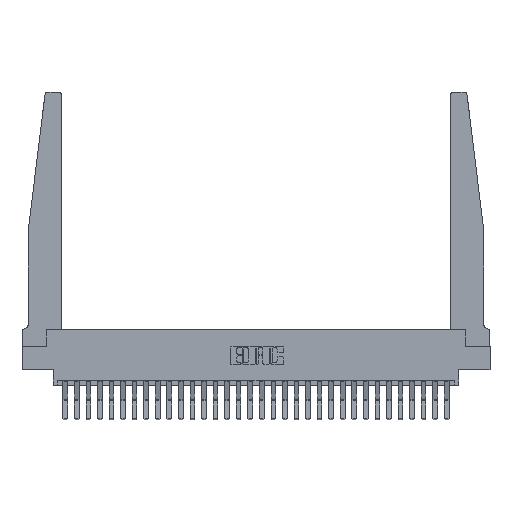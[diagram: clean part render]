
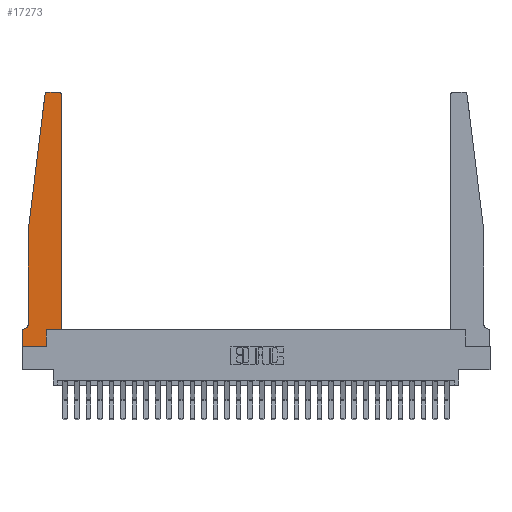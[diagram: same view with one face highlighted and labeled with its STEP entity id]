
A CAD part, top view. The second image highlights one B-rep face of the part: STEP entity #17273.
In plain terms, the highlighted planar face has unit normal (0, 0, 1).
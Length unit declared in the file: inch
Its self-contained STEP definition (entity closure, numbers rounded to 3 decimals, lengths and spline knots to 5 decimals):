
#343 = DIRECTION ( 'NONE',  ( 0., 0., 1. ) ) ;
#1655 = LINE ( 'NONE', #13245, #10600 ) ;
#1844 = LINE ( 'NONE', #19845, #6738 ) ;
#1891 = ORIENTED_EDGE ( 'NONE', *, *, #9325, .T. ) ;
#1930 = DIRECTION ( 'NONE',  ( 0., 0., 1. ) ) ;
#2151 = VERTEX_POINT ( 'NONE', #14245 ) ;
#2235 = VERTEX_POINT ( 'NONE', #6122 ) ;
#2693 = CARTESIAN_POINT ( 'NONE',  ( 0.2605, 0., 0.37 ) ) ;
#2800 = LINE ( 'NONE', #15864, #24524 ) ;
#2939 = CARTESIAN_POINT ( 'NONE',  ( 0.065, 1.25, 0.37 ) ) ;
#3071 = CARTESIAN_POINT ( 'NONE',  ( 0.395, 2.75, 0.37 ) ) ;
#3429 = VERTEX_POINT ( 'NONE', #3071 ) ;
#3630 = VECTOR ( 'NONE', #16445, 39.37008 ) ;
#4020 = EDGE_CURVE ( 'NONE', #3429, #2151, #14366, .T. ) ;
#4200 = CARTESIAN_POINT ( 'NONE',  ( 0.2605, 0.18, 0.37 ) ) ;
#4404 = DIRECTION ( 'NONE',  ( 0., -1., 0. ) ) ;
#4653 = VERTEX_POINT ( 'NONE', #10390 ) ;
#4699 = DIRECTION ( 'NONE',  ( 0., 1., 0. ) ) ;
#4990 = ORIENTED_EDGE ( 'NONE', *, *, #26933, .T. ) ;
#5367 = ORIENTED_EDGE ( 'NONE', *, *, #4020, .T. ) ;
#6033 = CARTESIAN_POINT ( 'NONE',  ( 0., 0.1875, 0.37 ) ) ;
#6117 = VECTOR ( 'NONE', #24935, 39.37008 ) ;
#6122 = CARTESIAN_POINT ( 'NONE',  ( 0., 0., 0.37 ) ) ;
#6321 = LINE ( 'NONE', #13255, #23984 ) ;
#6473 = CARTESIAN_POINT ( 'NONE',  ( 0.065, 0.1875, 0.37 ) ) ;
#6505 = VECTOR ( 'NONE', #15304, 39.37008 ) ;
#6738 = VECTOR ( 'NONE', #13789, 39.37008 ) ;
#6783 = LINE ( 'NONE', #18246, #6117 ) ;
#7001 = EDGE_CURVE ( 'NONE', #9190, #22807, #19394, .T. ) ;
#7300 = CARTESIAN_POINT ( 'NONE',  ( 0., 0., 0.37 ) ) ;
#7426 = DIRECTION ( 'NONE',  ( 0., 0., -1. ) ) ;
#7452 = DIRECTION ( 'NONE',  ( -0.122, -0.992, 0. ) ) ;
#7839 = DIRECTION ( 'NONE',  ( -1., 0., 0. ) ) ;
#8680 = CARTESIAN_POINT ( 'NONE',  ( 0.24675, 2.72367, 0.37 ) ) ;
#8735 = ORIENTED_EDGE ( 'NONE', *, *, #18170, .T. ) ;
#9190 = VERTEX_POINT ( 'NONE', #23740 ) ;
#9325 = EDGE_CURVE ( 'NONE', #10342, #4653, #6321, .T. ) ;
#10106 = CIRCLE ( 'NONE', #20796, 0.03 ) ;
#10124 = AXIS2_PLACEMENT_3D ( 'NONE', #12327, #16991, #25857 ) ;
#10177 = ORIENTED_EDGE ( 'NONE', *, *, #18561, .T. ) ;
#10342 = VERTEX_POINT ( 'NONE', #4200 ) ;
#10390 = CARTESIAN_POINT ( 'NONE',  ( 0.425, 0.18, 0.37 ) ) ;
#10600 = VECTOR ( 'NONE', #4404, 39.37008 ) ;
#11128 = VERTEX_POINT ( 'NONE', #6033 ) ;
#11210 = ORIENTED_EDGE ( 'NONE', *, *, #19764, .T. ) ;
#11516 = VERTEX_POINT ( 'NONE', #8680 ) ;
#11716 = VERTEX_POINT ( 'NONE', #16683 ) ;
#11878 = EDGE_CURVE ( 'NONE', #2235, #12019, #1844, .T. ) ;
#12019 = VERTEX_POINT ( 'NONE', #2693 ) ;
#12189 = DIRECTION ( 'NONE',  ( -1., 0., 0. ) ) ;
#12327 = CARTESIAN_POINT ( 'NONE',  ( 0., 0.1875, 0.37 ) ) ;
#13245 = CARTESIAN_POINT ( 'NONE',  ( 0.065, 1.25, 0.37 ) ) ;
#13255 = CARTESIAN_POINT ( 'NONE',  ( 0.425, 0.18, 0.37 ) ) ;
#13412 = DIRECTION ( 'NONE',  ( 1., 0., 0. ) ) ;
#13489 = VERTEX_POINT ( 'NONE', #23446 ) ;
#13789 = DIRECTION ( 'NONE',  ( 1., 0., 0. ) ) ;
#14245 = CARTESIAN_POINT ( 'NONE',  ( 0.27653, 2.75, 0.37 ) ) ;
#14366 = LINE ( 'NONE', #23229, #25247 ) ;
#14407 = ORIENTED_EDGE ( 'NONE', *, *, #18336, .T. ) ;
#14934 = FACE_OUTER_BOUND ( 'NONE', #23767, .T. ) ;
#15230 = EDGE_CURVE ( 'NONE', #2151, #11516, #10106, .T. ) ;
#15304 = DIRECTION ( 'NONE',  ( -1., 0., 0. ) ) ;
#15327 = EDGE_CURVE ( 'NONE', #11128, #2235, #27208, .T. ) ;
#15665 = AXIS2_PLACEMENT_3D ( 'NONE', #16124, #7426, #12189 ) ;
#15854 = CARTESIAN_POINT ( 'NONE',  ( 0.395, 2.72, 0.37 ) ) ;
#15864 = CARTESIAN_POINT ( 'NONE',  ( 0.2605, 0.18, 0.37 ) ) ;
#16124 = CARTESIAN_POINT ( 'NONE',  ( 0.015, 0.2375, 0.37 ) ) ;
#16445 = DIRECTION ( 'NONE',  ( 0., -1., 0. ) ) ;
#16451 = LINE ( 'NONE', #2939, #28271 ) ;
#16683 = CARTESIAN_POINT ( 'NONE',  ( 0.425, 2.72, 0.37 ) ) ;
#16991 = DIRECTION ( 'NONE',  ( 0., 0., 1. ) ) ;
#17273 = ADVANCED_FACE ( 'NONE', ( #14934 ), #19165, .T. ) ;
#17441 = ORIENTED_EDGE ( 'NONE', *, *, #7001, .T. ) ;
#17622 = DIRECTION ( 'NONE',  ( 1., 0., 0. ) ) ;
#18170 = EDGE_CURVE ( 'NONE', #13489, #9190, #1655, .T. ) ;
#18246 = CARTESIAN_POINT ( 'NONE',  ( 0.425, 0.18, 0.37 ) ) ;
#18336 = EDGE_CURVE ( 'NONE', #12019, #10342, #2800, .T. ) ;
#18561 = EDGE_CURVE ( 'NONE', #11516, #13489, #16451, .T. ) ;
#19165 = PLANE ( 'NONE',  #10124 ) ;
#19394 = CIRCLE ( 'NONE', #15665, 0.05 ) ;
#19469 = ORIENTED_EDGE ( 'NONE', *, *, #15327, .T. ) ;
#19764 = EDGE_CURVE ( 'NONE', #22807, #11128, #28554, .T. ) ;
#19845 = CARTESIAN_POINT ( 'NONE',  ( 0., 0., 0.37 ) ) ;
#20600 = AXIS2_PLACEMENT_3D ( 'NONE', #15854, #343, #22686 ) ;
#20796 = AXIS2_PLACEMENT_3D ( 'NONE', #21819, #1930, #17622 ) ;
#21819 = CARTESIAN_POINT ( 'NONE',  ( 0.27653, 2.72, 0.37 ) ) ;
#21941 = ORIENTED_EDGE ( 'NONE', *, *, #15230, .T. ) ;
#22686 = DIRECTION ( 'NONE',  ( 1., 0., 0. ) ) ;
#22807 = VERTEX_POINT ( 'NONE', #28679 ) ;
#23141 = EDGE_CURVE ( 'NONE', #4653, #11716, #6783, .T. ) ;
#23229 = CARTESIAN_POINT ( 'NONE',  ( 0.25, 2.75, 0.37 ) ) ;
#23446 = CARTESIAN_POINT ( 'NONE',  ( 0.065, 1.25, 0.37 ) ) ;
#23740 = CARTESIAN_POINT ( 'NONE',  ( 0.065, 0.2375, 0.37 ) ) ;
#23767 = EDGE_LOOP ( 'NONE', ( #5367, #21941, #10177, #8735, #17441, #11210, #19469, #27871, #14407, #1891, #24667, #4990 ) ) ;
#23984 = VECTOR ( 'NONE', #13412, 39.37008 ) ;
#24524 = VECTOR ( 'NONE', #4699, 39.37008 ) ;
#24667 = ORIENTED_EDGE ( 'NONE', *, *, #23141, .T. ) ;
#24935 = DIRECTION ( 'NONE',  ( 0., 1., 0. ) ) ;
#25247 = VECTOR ( 'NONE', #7839, 39.37008 ) ;
#25857 = DIRECTION ( 'NONE',  ( 1., 0., 0. ) ) ;
#26933 = EDGE_CURVE ( 'NONE', #11716, #3429, #27104, .T. ) ;
#27104 = CIRCLE ( 'NONE', #20600, 0.03 ) ;
#27208 = LINE ( 'NONE', #7300, #3630 ) ;
#27871 = ORIENTED_EDGE ( 'NONE', *, *, #11878, .T. ) ;
#28271 = VECTOR ( 'NONE', #7452, 39.37008 ) ;
#28554 = LINE ( 'NONE', #6473, #6505 ) ;
#28679 = CARTESIAN_POINT ( 'NONE',  ( 0.015, 0.1875, 0.37 ) ) ;
